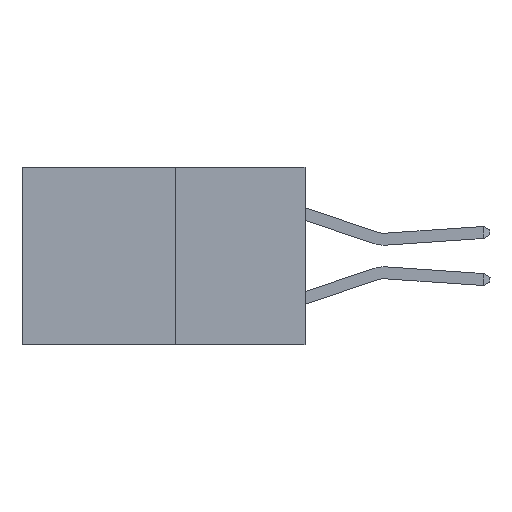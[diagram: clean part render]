
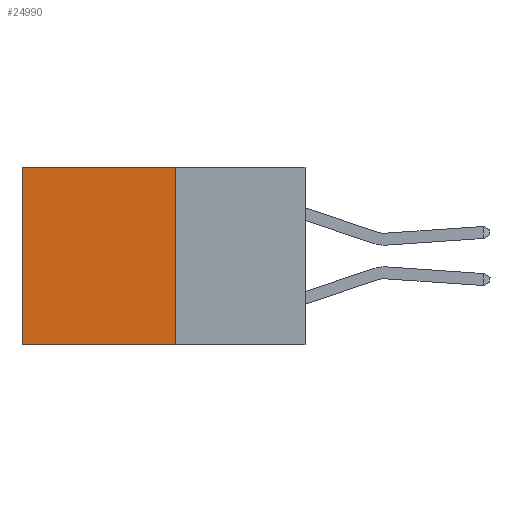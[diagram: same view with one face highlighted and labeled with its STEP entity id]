
A CAD part, left-side view. The second image highlights one B-rep face of the part: STEP entity #24990.
In plain terms, the highlighted planar face has unit normal (-1, 0, 0).
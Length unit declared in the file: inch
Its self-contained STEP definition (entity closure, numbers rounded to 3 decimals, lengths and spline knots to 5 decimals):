
#23 = CARTESIAN_POINT ( 'NONE',  ( 0.277, 0.59, -0.37 ) ) ;
#682 = CARTESIAN_POINT ( 'NONE',  ( 0.277, 0.27, -0.37 ) ) ;
#1154 = ORIENTED_EDGE ( 'NONE', *, *, #23588, .T. ) ;
#1475 = LINE ( 'NONE', #10885, #6834 ) ;
#1521 = DIRECTION ( 'NONE',  ( 0., 0., -1. ) ) ;
#1753 = FACE_OUTER_BOUND ( 'NONE', #18231, .T. ) ;
#4328 = EDGE_CURVE ( 'NONE', #20833, #13199, #18632, .T. ) ;
#4982 = LINE ( 'NONE', #23, #20468 ) ;
#5454 = EDGE_CURVE ( 'NONE', #20833, #6579, #17616, .T. ) ;
#5468 = EDGE_CURVE ( 'NONE', #13199, #9592, #1475, .T. ) ;
#5798 = ORIENTED_EDGE ( 'NONE', *, *, #5468, .F. ) ;
#6579 = VERTEX_POINT ( 'NONE', #22524 ) ;
#6593 = PLANE ( 'NONE',  #23484 ) ;
#6834 = VECTOR ( 'NONE', #23006, 39.37008 ) ;
#8448 = VECTOR ( 'NONE', #1521, 39.37008 ) ;
#8589 = DIRECTION ( 'NONE',  ( 0., 0., -1. ) ) ;
#9592 = VERTEX_POINT ( 'NONE', #22232 ) ;
#10552 = CARTESIAN_POINT ( 'NONE',  ( 0.277, 0.27, -0.37 ) ) ;
#10794 = CARTESIAN_POINT ( 'NONE',  ( 0.277, 0.27, 0. ) ) ;
#10885 = CARTESIAN_POINT ( 'NONE',  ( 0.277, 0.27, -0.37 ) ) ;
#11007 = CARTESIAN_POINT ( 'NONE',  ( 0.277, 0.27, 0. ) ) ;
#12214 = VECTOR ( 'NONE', #12850, 39.37008 ) ;
#12850 = DIRECTION ( 'NONE',  ( 0., 1., 0. ) ) ;
#13199 = VERTEX_POINT ( 'NONE', #682 ) ;
#15684 = CARTESIAN_POINT ( 'NONE',  ( 0.277, 0.27, -0.37 ) ) ;
#16243 = DIRECTION ( 'NONE',  ( 0., 0., -1. ) ) ;
#17616 = LINE ( 'NONE', #10794, #12214 ) ;
#18231 = EDGE_LOOP ( 'NONE', ( #1154, #5798, #21711, #18384 ) ) ;
#18384 = ORIENTED_EDGE ( 'NONE', *, *, #5454, .T. ) ;
#18632 = LINE ( 'NONE', #15684, #8448 ) ;
#20468 = VECTOR ( 'NONE', #16243, 39.37008 ) ;
#20731 = DIRECTION ( 'NONE',  ( 1., 0., 0. ) ) ;
#20833 = VERTEX_POINT ( 'NONE', #11007 ) ;
#21711 = ORIENTED_EDGE ( 'NONE', *, *, #4328, .F. ) ;
#22232 = CARTESIAN_POINT ( 'NONE',  ( 0.277, 0.59, -0.37 ) ) ;
#22524 = CARTESIAN_POINT ( 'NONE',  ( 0.277, 0.59, 0. ) ) ;
#23006 = DIRECTION ( 'NONE',  ( 0., 1., 0. ) ) ;
#23484 = AXIS2_PLACEMENT_3D ( 'NONE', #10552, #20731, #8589 ) ;
#23588 = EDGE_CURVE ( 'NONE', #6579, #9592, #4982, .T. ) ;
#24990 = ADVANCED_FACE ( 'NONE', ( #1753 ), #6593, .F. ) ;
